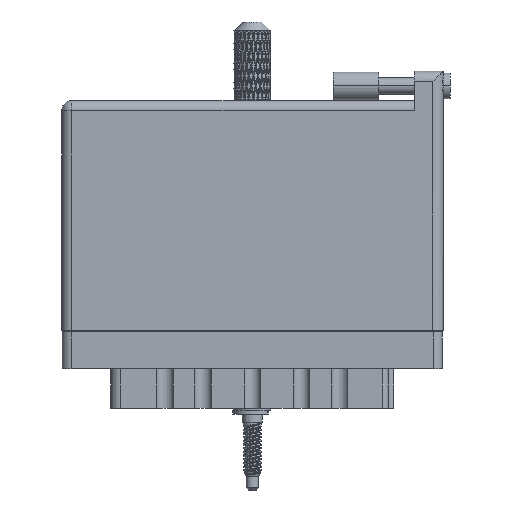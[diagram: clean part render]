
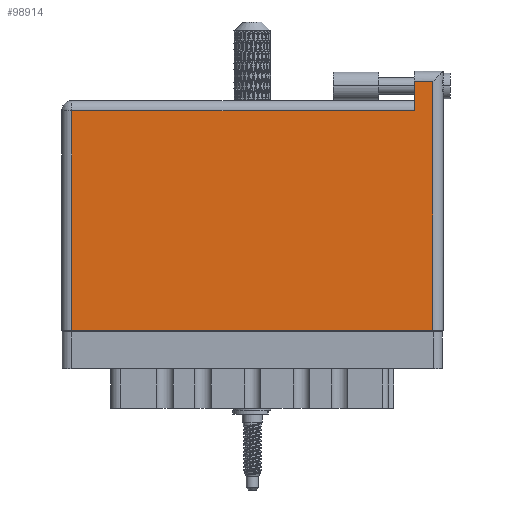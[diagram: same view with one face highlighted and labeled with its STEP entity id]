
A CAD part, front view. The second image highlights one B-rep face of the part: STEP entity #98914.
In plain terms, the highlighted face is planar.
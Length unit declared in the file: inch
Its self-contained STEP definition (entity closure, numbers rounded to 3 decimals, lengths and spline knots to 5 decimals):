
#47 = EDGE_CURVE ( 'NONE', #111462, #90162, #111876, .T. ) ;
#2426 = VECTOR ( 'NONE', #105556, 39.37008 ) ;
#5135 = DIRECTION ( 'NONE',  ( -1., 0., 0. ) ) ;
#8514 = CARTESIAN_POINT ( 'NONE',  ( 2.53, 1.696, 0. ) ) ;
#10186 = ORIENTED_EDGE ( 'NONE', *, *, #105856, .T. ) ;
#12309 = ORIENTED_EDGE ( 'NONE', *, *, #67782, .T. ) ;
#14365 = EDGE_CURVE ( 'NONE', #112807, #110891, #67550, .T. ) ;
#15471 = CARTESIAN_POINT ( 'NONE',  ( 2.403, 1.696, 0. ) ) ;
#16597 = VECTOR ( 'NONE', #5135, 39.37008 ) ;
#17829 = ORIENTED_EDGE ( 'NONE', *, *, #21782, .T. ) ;
#18144 = VECTOR ( 'NONE', #63196, 39.37008 ) ;
#21782 = EDGE_CURVE ( 'NONE', #110891, #31767, #44416, .T. ) ;
#25093 = CARTESIAN_POINT ( 'NONE',  ( 2.403, 1.766, 0. ) ) ;
#27220 = CARTESIAN_POINT ( 'NONE',  ( 0.07, 0., 0. ) ) ;
#30822 = CARTESIAN_POINT ( 'NONE',  ( 0.07, 0., 0. ) ) ;
#31712 = CARTESIAN_POINT ( 'NONE',  ( 2.403, 1.496, 0. ) ) ;
#31767 = VERTEX_POINT ( 'NONE', #46975 ) ;
#32551 = EDGE_CURVE ( 'NONE', #84560, #111462, #113189, .T. ) ;
#34509 = ORIENTED_EDGE ( 'NONE', *, *, #47, .T. ) ;
#41388 = EDGE_LOOP ( 'NONE', ( #48682, #34509, #12309, #78991, #17829, #10186 ) ) ;
#44416 = LINE ( 'NONE', #112319, #16597 ) ;
#46975 = CARTESIAN_POINT ( 'NONE',  ( 0.07, 1.496, 0. ) ) ;
#48682 = ORIENTED_EDGE ( 'NONE', *, *, #32551, .T. ) ;
#52552 = CARTESIAN_POINT ( 'NONE',  ( 2.53, 0., 0. ) ) ;
#55045 = VECTOR ( 'NONE', #74667, 39.37008 ) ;
#59748 = LINE ( 'NONE', #106797, #18144 ) ;
#63196 = DIRECTION ( 'NONE',  ( -1., 0., 0. ) ) ;
#64919 = VECTOR ( 'NONE', #106438, 39.37008 ) ;
#67550 = LINE ( 'NONE', #25093, #2426 ) ;
#67782 = EDGE_CURVE ( 'NONE', #90162, #112807, #59748, .T. ) ;
#70771 = FACE_OUTER_BOUND ( 'NONE', #41388, .T. ) ;
#71724 = CARTESIAN_POINT ( 'NONE',  ( 2.53, 1.766, 0. ) ) ;
#74667 = DIRECTION ( 'NONE',  ( 0., -1., 0. ) ) ;
#77297 = VECTOR ( 'NONE', #108222, 39.37008 ) ;
#78625 = CARTESIAN_POINT ( 'NONE',  ( 0., 1.566, 0. ) ) ;
#78991 = ORIENTED_EDGE ( 'NONE', *, *, #14365, .T. ) ;
#84560 = VERTEX_POINT ( 'NONE', #27220 ) ;
#87768 = AXIS2_PLACEMENT_3D ( 'NONE', #78625, #105203, #87868 ) ;
#87868 = DIRECTION ( 'NONE',  ( -1., 0., 0. ) ) ;
#90162 = VERTEX_POINT ( 'NONE', #8514 ) ;
#90565 = CARTESIAN_POINT ( 'NONE',  ( 0., 0., 0. ) ) ;
#93654 = LINE ( 'NONE', #30822, #55045 ) ;
#98914 = ADVANCED_FACE ( 'NONE', ( #70771 ), #105585, .F. ) ;
#105203 = DIRECTION ( 'NONE',  ( 0., 0., -1. ) ) ;
#105556 = DIRECTION ( 'NONE',  ( 0., -1., 0. ) ) ;
#105585 = PLANE ( 'NONE',  #87768 ) ;
#105856 = EDGE_CURVE ( 'NONE', #31767, #84560, #93654, .T. ) ;
#106438 = DIRECTION ( 'NONE',  ( 0., 1., 0. ) ) ;
#106797 = CARTESIAN_POINT ( 'NONE',  ( 0., 1.696, 0. ) ) ;
#108222 = DIRECTION ( 'NONE',  ( 1., 0., 0. ) ) ;
#110891 = VERTEX_POINT ( 'NONE', #31712 ) ;
#111462 = VERTEX_POINT ( 'NONE', #52552 ) ;
#111876 = LINE ( 'NONE', #71724, #64919 ) ;
#112319 = CARTESIAN_POINT ( 'NONE',  ( 0., 1.496, 0. ) ) ;
#112807 = VERTEX_POINT ( 'NONE', #15471 ) ;
#113189 = LINE ( 'NONE', #90565, #77297 ) ;
